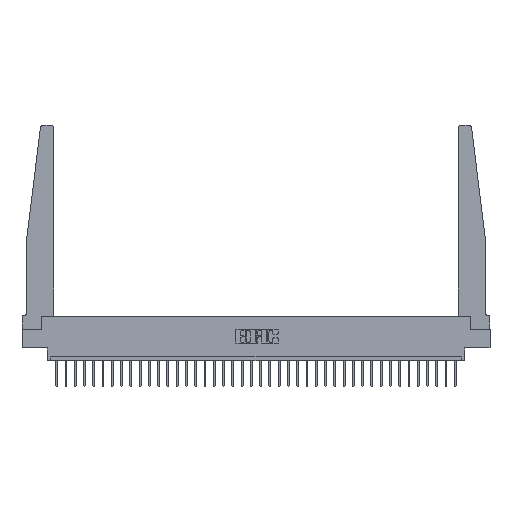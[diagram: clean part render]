
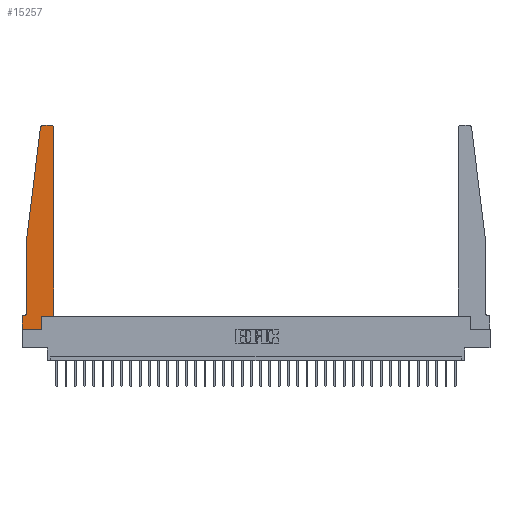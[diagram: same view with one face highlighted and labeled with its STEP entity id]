
A CAD part, top view. The second image highlights one B-rep face of the part: STEP entity #15257.
In plain terms, the highlighted planar face has unit normal (0, 0, 1).
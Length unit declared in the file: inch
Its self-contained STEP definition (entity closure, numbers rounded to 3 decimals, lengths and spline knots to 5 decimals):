
#104 = CARTESIAN_POINT ( 'NONE',  ( 0.395, 2.75, 0.37 ) ) ;
#639 = CARTESIAN_POINT ( 'NONE',  ( 0.425, 0.18, 0.37 ) ) ;
#1118 = EDGE_CURVE ( 'NONE', #6932, #22983, #25267, .T. ) ;
#1148 = VECTOR ( 'NONE', #11864, 39.37008 ) ;
#1593 = EDGE_CURVE ( 'NONE', #23747, #22737, #16771, .T. ) ;
#2439 = DIRECTION ( 'NONE',  ( -1., 0., 0. ) ) ;
#2520 = CARTESIAN_POINT ( 'NONE',  ( 0.2605, 0., 0.37 ) ) ;
#2782 = CARTESIAN_POINT ( 'NONE',  ( 0., 0.1875, 0.37 ) ) ;
#2838 = CARTESIAN_POINT ( 'NONE',  ( 0.015, 0.2375, 0.37 ) ) ;
#3329 = CARTESIAN_POINT ( 'NONE',  ( 0.065, 1.25, 0.37 ) ) ;
#3670 = EDGE_CURVE ( 'NONE', #30310, #23747, #6593, .T. ) ;
#3842 = CARTESIAN_POINT ( 'NONE',  ( 0.2605, 0.18, 0.37 ) ) ;
#4514 = DIRECTION ( 'NONE',  ( 1., 0., 0. ) ) ;
#5113 = DIRECTION ( 'NONE',  ( -1., 0., 0. ) ) ;
#5194 = DIRECTION ( 'NONE',  ( 1., 0., 0. ) ) ;
#5577 = CARTESIAN_POINT ( 'NONE',  ( 0.24675, 2.72367, 0.37 ) ) ;
#5591 = EDGE_CURVE ( 'NONE', #10610, #30003, #19196, .T. ) ;
#5606 = DIRECTION ( 'NONE',  ( -0.122, -0.992, 0. ) ) ;
#5786 = ORIENTED_EDGE ( 'NONE', *, *, #19880, .T. ) ;
#5818 = VECTOR ( 'NONE', #26153, 39.37008 ) ;
#5905 = CARTESIAN_POINT ( 'NONE',  ( 0.27653, 2.75, 0.37 ) ) ;
#6593 = LINE ( 'NONE', #26381, #1148 ) ;
#6736 = VECTOR ( 'NONE', #25145, 39.37008 ) ;
#6831 = EDGE_CURVE ( 'NONE', #11506, #30310, #16439, .T. ) ;
#6932 = VERTEX_POINT ( 'NONE', #8913 ) ;
#7077 = VECTOR ( 'NONE', #12861, 39.37008 ) ;
#7247 = CARTESIAN_POINT ( 'NONE',  ( 0., 0., 0.37 ) ) ;
#7854 = CARTESIAN_POINT ( 'NONE',  ( 0.425, 0.18, 0.37 ) ) ;
#7855 = ORIENTED_EDGE ( 'NONE', *, *, #11588, .T. ) ;
#8110 = ORIENTED_EDGE ( 'NONE', *, *, #30588, .T. ) ;
#8869 = CIRCLE ( 'NONE', #9597, 0.03 ) ;
#8913 = CARTESIAN_POINT ( 'NONE',  ( 0.425, 0.18, 0.37 ) ) ;
#8935 = LINE ( 'NONE', #18225, #30183 ) ;
#9431 = EDGE_CURVE ( 'NONE', #15658, #6932, #19073, .T. ) ;
#9597 = AXIS2_PLACEMENT_3D ( 'NONE', #10464, #24997, #17994 ) ;
#10464 = CARTESIAN_POINT ( 'NONE',  ( 0.395, 2.72, 0.37 ) ) ;
#10499 = LINE ( 'NONE', #31330, #11283 ) ;
#10610 = VERTEX_POINT ( 'NONE', #5905 ) ;
#11178 = CIRCLE ( 'NONE', #12315, 0.05 ) ;
#11274 = ORIENTED_EDGE ( 'NONE', *, *, #5591, .T. ) ;
#11283 = VECTOR ( 'NONE', #16564, 39.37008 ) ;
#11332 = CARTESIAN_POINT ( 'NONE',  ( 0.015, 0.1875, 0.37 ) ) ;
#11506 = VERTEX_POINT ( 'NONE', #11332 ) ;
#11588 = EDGE_CURVE ( 'NONE', #18832, #10610, #10499, .T. ) ;
#11864 = DIRECTION ( 'NONE',  ( 0., -1., 0. ) ) ;
#12217 = CARTESIAN_POINT ( 'NONE',  ( 0., 0., 0.37 ) ) ;
#12315 = AXIS2_PLACEMENT_3D ( 'NONE', #2838, #29920, #5113 ) ;
#12599 = ORIENTED_EDGE ( 'NONE', *, *, #20665, .T. ) ;
#12861 = DIRECTION ( 'NONE',  ( 1., 0., 0. ) ) ;
#12870 = CARTESIAN_POINT ( 'NONE',  ( 0.065, 1.25, 0.37 ) ) ;
#13108 = FACE_OUTER_BOUND ( 'NONE', #27396, .T. ) ;
#13804 = VERTEX_POINT ( 'NONE', #28254 ) ;
#13888 = ORIENTED_EDGE ( 'NONE', *, *, #29967, .T. ) ;
#14385 = LINE ( 'NONE', #3329, #29070 ) ;
#14730 = PLANE ( 'NONE',  #31815 ) ;
#14838 = DIRECTION ( 'NONE',  ( 1., 0., 0. ) ) ;
#15257 = ADVANCED_FACE ( 'NONE', ( #13108 ), #14730, .T. ) ;
#15297 = ORIENTED_EDGE ( 'NONE', *, *, #6831, .T. ) ;
#15658 = VERTEX_POINT ( 'NONE', #22667 ) ;
#16439 = LINE ( 'NONE', #17579, #19505 ) ;
#16564 = DIRECTION ( 'NONE',  ( -1., 0., 0. ) ) ;
#16771 = LINE ( 'NONE', #7247, #29467 ) ;
#17579 = CARTESIAN_POINT ( 'NONE',  ( 0.065, 0.1875, 0.37 ) ) ;
#17994 = DIRECTION ( 'NONE',  ( 1., 0., 0. ) ) ;
#18225 = CARTESIAN_POINT ( 'NONE',  ( 0.065, 1.25, 0.37 ) ) ;
#18309 = EDGE_CURVE ( 'NONE', #30003, #29449, #14385, .T. ) ;
#18832 = VERTEX_POINT ( 'NONE', #104 ) ;
#19073 = LINE ( 'NONE', #7854, #7077 ) ;
#19196 = CIRCLE ( 'NONE', #21208, 0.03 ) ;
#19505 = VECTOR ( 'NONE', #2439, 39.37008 ) ;
#19880 = EDGE_CURVE ( 'NONE', #29449, #13804, #8935, .T. ) ;
#19909 = DIRECTION ( 'NONE',  ( 0., 0., 1. ) ) ;
#20084 = ORIENTED_EDGE ( 'NONE', *, *, #1593, .T. ) ;
#20665 = EDGE_CURVE ( 'NONE', #22737, #15658, #29018, .T. ) ;
#20895 = DIRECTION ( 'NONE',  ( 0., 0., 1. ) ) ;
#21208 = AXIS2_PLACEMENT_3D ( 'NONE', #30217, #20895, #4514 ) ;
#21390 = CARTESIAN_POINT ( 'NONE',  ( 0., 0.1875, 0.37 ) ) ;
#22667 = CARTESIAN_POINT ( 'NONE',  ( 0.2605, 0.18, 0.37 ) ) ;
#22737 = VERTEX_POINT ( 'NONE', #2520 ) ;
#22983 = VERTEX_POINT ( 'NONE', #25722 ) ;
#23167 = DIRECTION ( 'NONE',  ( 0., -1., 0. ) ) ;
#23379 = ORIENTED_EDGE ( 'NONE', *, *, #3670, .T. ) ;
#23723 = ORIENTED_EDGE ( 'NONE', *, *, #9431, .T. ) ;
#23747 = VERTEX_POINT ( 'NONE', #12217 ) ;
#24902 = ORIENTED_EDGE ( 'NONE', *, *, #1118, .T. ) ;
#24997 = DIRECTION ( 'NONE',  ( 0., 0., 1. ) ) ;
#25145 = DIRECTION ( 'NONE',  ( 0., 1., 0. ) ) ;
#25267 = LINE ( 'NONE', #639, #6736 ) ;
#25722 = CARTESIAN_POINT ( 'NONE',  ( 0.425, 2.72, 0.37 ) ) ;
#26153 = DIRECTION ( 'NONE',  ( 0., 1., 0. ) ) ;
#26381 = CARTESIAN_POINT ( 'NONE',  ( 0., 0., 0.37 ) ) ;
#27301 = ORIENTED_EDGE ( 'NONE', *, *, #18309, .T. ) ;
#27396 = EDGE_LOOP ( 'NONE', ( #7855, #11274, #27301, #5786, #8110, #15297, #23379, #20084, #12599, #23723, #24902, #13888 ) ) ;
#28254 = CARTESIAN_POINT ( 'NONE',  ( 0.065, 0.2375, 0.37 ) ) ;
#29018 = LINE ( 'NONE', #3842, #5818 ) ;
#29070 = VECTOR ( 'NONE', #5606, 39.37008 ) ;
#29449 = VERTEX_POINT ( 'NONE', #12870 ) ;
#29467 = VECTOR ( 'NONE', #5194, 39.37008 ) ;
#29920 = DIRECTION ( 'NONE',  ( 0., 0., -1. ) ) ;
#29967 = EDGE_CURVE ( 'NONE', #22983, #18832, #8869, .T. ) ;
#30003 = VERTEX_POINT ( 'NONE', #5577 ) ;
#30183 = VECTOR ( 'NONE', #23167, 39.37008 ) ;
#30217 = CARTESIAN_POINT ( 'NONE',  ( 0.27653, 2.72, 0.37 ) ) ;
#30310 = VERTEX_POINT ( 'NONE', #21390 ) ;
#30588 = EDGE_CURVE ( 'NONE', #13804, #11506, #11178, .T. ) ;
#31330 = CARTESIAN_POINT ( 'NONE',  ( 0.25, 2.75, 0.37 ) ) ;
#31815 = AXIS2_PLACEMENT_3D ( 'NONE', #2782, #19909, #14838 ) ;
